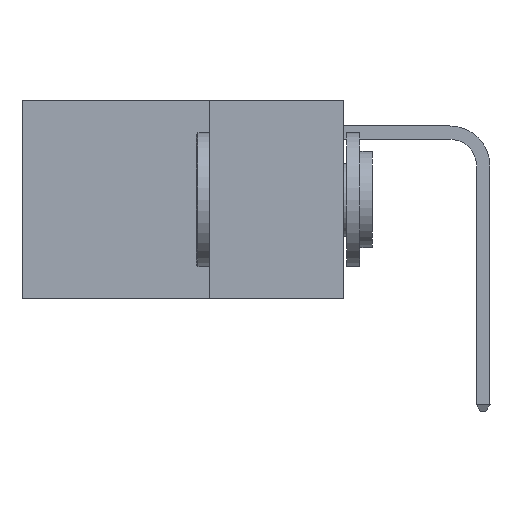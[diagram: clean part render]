
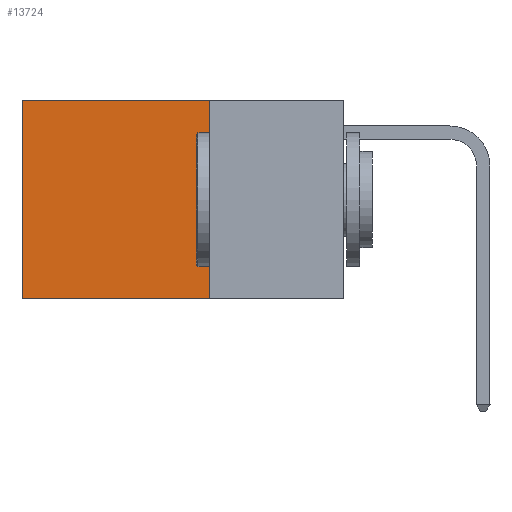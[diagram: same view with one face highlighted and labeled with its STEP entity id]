
A CAD part, left-side view. The second image highlights one B-rep face of the part: STEP entity #13724.
In plain terms, the highlighted planar face has unit normal (-1, 0, 0).
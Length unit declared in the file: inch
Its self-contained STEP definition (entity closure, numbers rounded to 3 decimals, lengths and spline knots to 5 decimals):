
#987 = PLANE ( 'NONE',  #27594 ) ;
#1112 = DIRECTION ( 'NONE',  ( 1., 0., 0. ) ) ;
#4351 = LINE ( 'NONE', #12788, #6463 ) ;
#6463 = VECTOR ( 'NONE', #19394, 39.37008 ) ;
#6894 = VERTEX_POINT ( 'NONE', #22830 ) ;
#7437 = CARTESIAN_POINT ( 'NONE',  ( 0.2625, 0.25, 0. ) ) ;
#9589 = CARTESIAN_POINT ( 'NONE',  ( 0.2625, 0.6, 0. ) ) ;
#10390 = ORIENTED_EDGE ( 'NONE', *, *, #25988, .F. ) ;
#12788 = CARTESIAN_POINT ( 'NONE',  ( 0.2625, 0.25, -0.37 ) ) ;
#13013 = CARTESIAN_POINT ( 'NONE',  ( 0.2625, 0.25, -0.37 ) ) ;
#13333 = EDGE_CURVE ( 'NONE', #6894, #25911, #24598, .T. ) ;
#13389 = ORIENTED_EDGE ( 'NONE', *, *, #24432, .T. ) ;
#13724 = ADVANCED_FACE ( 'NONE', ( #26536 ), #987, .F. ) ;
#14063 = ORIENTED_EDGE ( 'NONE', *, *, #20784, .F. ) ;
#14466 = VERTEX_POINT ( 'NONE', #13013 ) ;
#14501 = CARTESIAN_POINT ( 'NONE',  ( 0.2625, 0.25, 0. ) ) ;
#16228 = ORIENTED_EDGE ( 'NONE', *, *, #13333, .T. ) ;
#17276 = VECTOR ( 'NONE', #18025, 39.37008 ) ;
#17406 = CARTESIAN_POINT ( 'NONE',  ( 0.2625, 0.25, 0. ) ) ;
#17817 = VECTOR ( 'NONE', #23568, 39.37008 ) ;
#18025 = DIRECTION ( 'NONE',  ( 0., 0., -1. ) ) ;
#19394 = DIRECTION ( 'NONE',  ( 0., 1., 0. ) ) ;
#20208 = LINE ( 'NONE', #17406, #24178 ) ;
#20784 = EDGE_CURVE ( 'NONE', #14466, #25911, #4351, .T. ) ;
#21735 = EDGE_LOOP ( 'NONE', ( #16228, #14063, #10390, #13389 ) ) ;
#21878 = DIRECTION ( 'NONE',  ( 0., 0., -1. ) ) ;
#22188 = DIRECTION ( 'NONE',  ( 0., 0., -1. ) ) ;
#22830 = CARTESIAN_POINT ( 'NONE',  ( 0.2625, 0.6, 0. ) ) ;
#23568 = DIRECTION ( 'NONE',  ( 0., 1., 0. ) ) ;
#24178 = VECTOR ( 'NONE', #21878, 39.37008 ) ;
#24432 = EDGE_CURVE ( 'NONE', #26010, #6894, #25300, .T. ) ;
#24598 = LINE ( 'NONE', #9589, #17276 ) ;
#25300 = LINE ( 'NONE', #14501, #17817 ) ;
#25911 = VERTEX_POINT ( 'NONE', #26509 ) ;
#25958 = CARTESIAN_POINT ( 'NONE',  ( 0.2625, 0.25, 0. ) ) ;
#25988 = EDGE_CURVE ( 'NONE', #26010, #14466, #20208, .T. ) ;
#26010 = VERTEX_POINT ( 'NONE', #25958 ) ;
#26509 = CARTESIAN_POINT ( 'NONE',  ( 0.2625, 0.6, -0.37 ) ) ;
#26536 = FACE_OUTER_BOUND ( 'NONE', #21735, .T. ) ;
#27594 = AXIS2_PLACEMENT_3D ( 'NONE', #7437, #1112, #22188 ) ;
